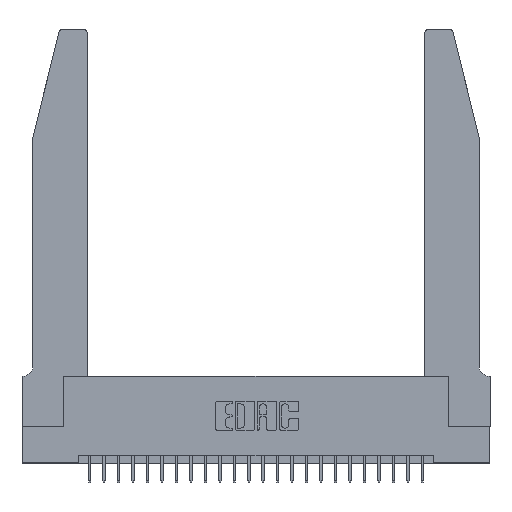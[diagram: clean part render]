
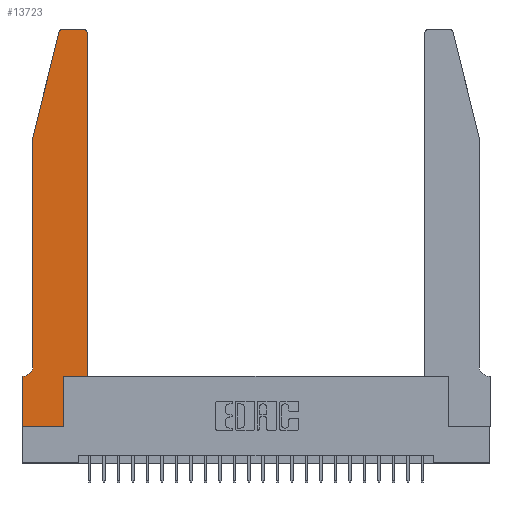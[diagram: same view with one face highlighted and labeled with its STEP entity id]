
A CAD part, top view. The second image highlights one B-rep face of the part: STEP entity #13723.
In plain terms, the highlighted planar face has unit normal (0, 0, 1).
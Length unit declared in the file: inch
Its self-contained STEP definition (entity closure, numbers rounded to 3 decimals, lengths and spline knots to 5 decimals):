
#149 = DIRECTION ( 'NONE',  ( -1., 0., 0. ) ) ;
#899 = VERTEX_POINT ( 'NONE', #15562 ) ;
#1466 = ORIENTED_EDGE ( 'NONE', *, *, #22736, .T. ) ;
#1652 = DIRECTION ( 'NONE',  ( 0., 0., 1. ) ) ;
#1736 = PLANE ( 'NONE',  #17763 ) ;
#2146 = CARTESIAN_POINT ( 'NONE',  ( 0.25487, 2.72718, 0.37 ) ) ;
#2203 = DIRECTION ( 'NONE',  ( 0., 1., 0. ) ) ;
#2552 = CARTESIAN_POINT ( 'NONE',  ( 0.284, 2.75, 0.37 ) ) ;
#2672 = DIRECTION ( 'NONE',  ( -0.239, -0.971, 0. ) ) ;
#2792 = VERTEX_POINT ( 'NONE', #2146 ) ;
#3357 = DIRECTION ( 'NONE',  ( 1., 0., 0. ) ) ;
#3942 = VERTEX_POINT ( 'NONE', #14683 ) ;
#4742 = VERTEX_POINT ( 'NONE', #20033 ) ;
#5178 = LINE ( 'NONE', #13256, #9104 ) ;
#5255 = AXIS2_PLACEMENT_3D ( 'NONE', #7323, #11545, #3357 ) ;
#5364 = CARTESIAN_POINT ( 'NONE',  ( 0.4505, 2.72, 0.37 ) ) ;
#5461 = CARTESIAN_POINT ( 'NONE',  ( 0., 0.35, 0.37 ) ) ;
#5587 = EDGE_LOOP ( 'NONE', ( #19556, #9244, #17266, #10647, #7175, #22400, #13758, #24823, #6959, #1466, #19264, #18792 ) ) ;
#6279 = EDGE_CURVE ( 'NONE', #9704, #2792, #6960, .T. ) ;
#6413 = CARTESIAN_POINT ( 'NONE',  ( 0.2865, 0., 0.37 ) ) ;
#6744 = EDGE_CURVE ( 'NONE', #24075, #22761, #5178, .T. ) ;
#6959 = ORIENTED_EDGE ( 'NONE', *, *, #7695, .T. ) ;
#6960 = CIRCLE ( 'NONE', #5255, 0.03 ) ;
#7040 = EDGE_CURVE ( 'NONE', #899, #23662, #8468, .T. ) ;
#7175 = ORIENTED_EDGE ( 'NONE', *, *, #21939, .T. ) ;
#7323 = CARTESIAN_POINT ( 'NONE',  ( 0.284, 2.72, 0.37 ) ) ;
#7520 = CARTESIAN_POINT ( 'NONE',  ( 0.2865, 0.35, 0.37 ) ) ;
#7695 = EDGE_CURVE ( 'NONE', #22761, #18646, #9503, .T. ) ;
#7742 = CARTESIAN_POINT ( 'NONE',  ( 0.0755, 0.35, 0.37 ) ) ;
#7865 = AXIS2_PLACEMENT_3D ( 'NONE', #20776, #12465, #149 ) ;
#8220 = EDGE_CURVE ( 'NONE', #9585, #3942, #14093, .T. ) ;
#8312 = VECTOR ( 'NONE', #10243, 39.37008 ) ;
#8468 = LINE ( 'NONE', #10458, #18796 ) ;
#8487 = CARTESIAN_POINT ( 'NONE',  ( 0.2865, 0.35, 0.37 ) ) ;
#8500 = EDGE_CURVE ( 'NONE', #2792, #899, #16704, .T. ) ;
#8679 = LINE ( 'NONE', #10798, #15273 ) ;
#9104 = VECTOR ( 'NONE', #19446, 39.37008 ) ;
#9244 = ORIENTED_EDGE ( 'NONE', *, *, #6279, .T. ) ;
#9503 = LINE ( 'NONE', #7520, #24310 ) ;
#9585 = VERTEX_POINT ( 'NONE', #18038 ) ;
#9704 = VERTEX_POINT ( 'NONE', #2552 ) ;
#10149 = DIRECTION ( 'NONE',  ( -1., 0., 0. ) ) ;
#10243 = DIRECTION ( 'NONE',  ( -1., 0., 0. ) ) ;
#10458 = CARTESIAN_POINT ( 'NONE',  ( 0.0755, 2., 0.37 ) ) ;
#10647 = ORIENTED_EDGE ( 'NONE', *, *, #7040, .T. ) ;
#10798 = CARTESIAN_POINT ( 'NONE',  ( 0., 0., 0.37 ) ) ;
#10825 = CARTESIAN_POINT ( 'NONE',  ( 0., 0., 0.37 ) ) ;
#11531 = AXIS2_PLACEMENT_3D ( 'NONE', #19635, #1652, #23845 ) ;
#11545 = DIRECTION ( 'NONE',  ( 0., 0., 1. ) ) ;
#12465 = DIRECTION ( 'NONE',  ( 0., 0., -1. ) ) ;
#12503 = DIRECTION ( 'NONE',  ( 1., 0., 0. ) ) ;
#13256 = CARTESIAN_POINT ( 'NONE',  ( 0., 0., 0.37 ) ) ;
#13723 = ADVANCED_FACE ( 'NONE', ( #19592 ), #1736, .T. ) ;
#13758 = ORIENTED_EDGE ( 'NONE', *, *, #15455, .T. ) ;
#14093 = LINE ( 'NONE', #7742, #8312 ) ;
#14210 = VECTOR ( 'NONE', #12503, 39.37008 ) ;
#14683 = CARTESIAN_POINT ( 'NONE',  ( 0., 0.35, 0.37 ) ) ;
#15273 = VECTOR ( 'NONE', #18320, 39.37008 ) ;
#15455 = EDGE_CURVE ( 'NONE', #3942, #24075, #8679, .T. ) ;
#15562 = CARTESIAN_POINT ( 'NONE',  ( 0.0755, 2., 0.37 ) ) ;
#16012 = DIRECTION ( 'NONE',  ( 0., 0., 1. ) ) ;
#16085 = LINE ( 'NONE', #22178, #21280 ) ;
#16159 = CIRCLE ( 'NONE', #11531, 0.03 ) ;
#16276 = CIRCLE ( 'NONE', #7865, 0.07 ) ;
#16704 = LINE ( 'NONE', #24755, #18429 ) ;
#16886 = EDGE_CURVE ( 'NONE', #19953, #4742, #16159, .T. ) ;
#17266 = ORIENTED_EDGE ( 'NONE', *, *, #8500, .T. ) ;
#17707 = VECTOR ( 'NONE', #10149, 39.37008 ) ;
#17762 = EDGE_CURVE ( 'NONE', #22997, #19953, #16085, .T. ) ;
#17763 = AXIS2_PLACEMENT_3D ( 'NONE', #5461, #16012, #24071 ) ;
#18038 = CARTESIAN_POINT ( 'NONE',  ( 0.0055, 0.35, 0.37 ) ) ;
#18320 = DIRECTION ( 'NONE',  ( 0., -1., 0. ) ) ;
#18429 = VECTOR ( 'NONE', #2672, 39.37008 ) ;
#18574 = CARTESIAN_POINT ( 'NONE',  ( 0.4505, 0.35, 0.37 ) ) ;
#18646 = VERTEX_POINT ( 'NONE', #8487 ) ;
#18792 = ORIENTED_EDGE ( 'NONE', *, *, #16886, .T. ) ;
#18796 = VECTOR ( 'NONE', #22348, 39.37008 ) ;
#19264 = ORIENTED_EDGE ( 'NONE', *, *, #17762, .T. ) ;
#19446 = DIRECTION ( 'NONE',  ( 1., 0., 0. ) ) ;
#19556 = ORIENTED_EDGE ( 'NONE', *, *, #25696, .T. ) ;
#19592 = FACE_OUTER_BOUND ( 'NONE', #5587, .T. ) ;
#19635 = CARTESIAN_POINT ( 'NONE',  ( 0.4205, 2.72, 0.37 ) ) ;
#19953 = VERTEX_POINT ( 'NONE', #5364 ) ;
#20033 = CARTESIAN_POINT ( 'NONE',  ( 0.4205, 2.75, 0.37 ) ) ;
#20314 = CARTESIAN_POINT ( 'NONE',  ( 0.2605, 2.75, 0.37 ) ) ;
#20776 = CARTESIAN_POINT ( 'NONE',  ( 0.0055, 0.42, 0.37 ) ) ;
#20886 = CARTESIAN_POINT ( 'NONE',  ( 0.0755, 0.42, 0.37 ) ) ;
#21280 = VECTOR ( 'NONE', #2203, 39.37008 ) ;
#21939 = EDGE_CURVE ( 'NONE', #23662, #9585, #16276, .T. ) ;
#22178 = CARTESIAN_POINT ( 'NONE',  ( 0.4505, 0.35, 0.37 ) ) ;
#22348 = DIRECTION ( 'NONE',  ( 0., -1., 0. ) ) ;
#22400 = ORIENTED_EDGE ( 'NONE', *, *, #8220, .T. ) ;
#22736 = EDGE_CURVE ( 'NONE', #18646, #22997, #22791, .T. ) ;
#22761 = VERTEX_POINT ( 'NONE', #6413 ) ;
#22791 = LINE ( 'NONE', #18574, #14210 ) ;
#22997 = VERTEX_POINT ( 'NONE', #23960 ) ;
#23620 = DIRECTION ( 'NONE',  ( 0., 1., 0. ) ) ;
#23662 = VERTEX_POINT ( 'NONE', #20886 ) ;
#23845 = DIRECTION ( 'NONE',  ( 1., 0., 0. ) ) ;
#23960 = CARTESIAN_POINT ( 'NONE',  ( 0.4505, 0.35, 0.37 ) ) ;
#24071 = DIRECTION ( 'NONE',  ( 1., 0., 0. ) ) ;
#24075 = VERTEX_POINT ( 'NONE', #10825 ) ;
#24267 = LINE ( 'NONE', #20314, #17707 ) ;
#24310 = VECTOR ( 'NONE', #23620, 39.37008 ) ;
#24755 = CARTESIAN_POINT ( 'NONE',  ( 0.0755, 2., 0.37 ) ) ;
#24823 = ORIENTED_EDGE ( 'NONE', *, *, #6744, .T. ) ;
#25696 = EDGE_CURVE ( 'NONE', #4742, #9704, #24267, .T. ) ;
